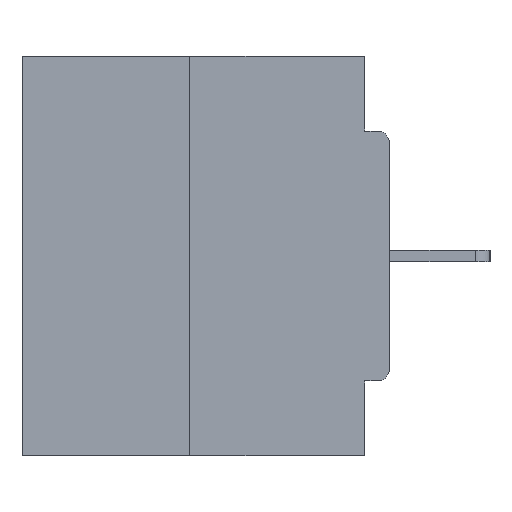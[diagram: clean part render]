
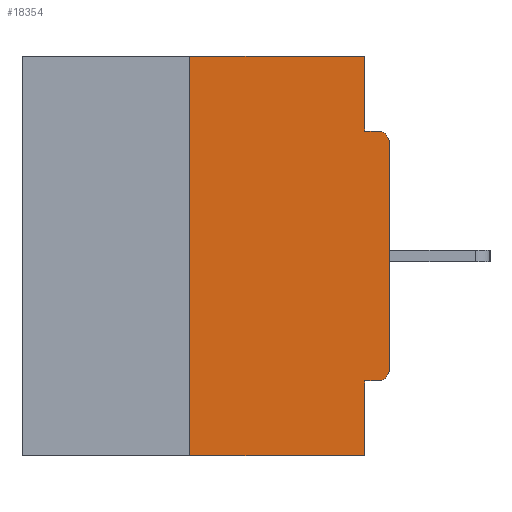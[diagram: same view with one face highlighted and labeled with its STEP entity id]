
A CAD part, left-side view. The second image highlights one B-rep face of the part: STEP entity #18354.
In plain terms, the highlighted planar face has unit normal (-1, 0, 0).
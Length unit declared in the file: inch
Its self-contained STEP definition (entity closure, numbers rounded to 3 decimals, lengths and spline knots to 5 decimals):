
#878 = CARTESIAN_POINT ( 'NONE',  ( 0., 0.25, -0.5 ) ) ;
#1514 = VERTEX_POINT ( 'NONE', #3295 ) ;
#1581 = VECTOR ( 'NONE', #13170, 39.37008 ) ;
#1629 = CARTESIAN_POINT ( 'NONE',  ( 0., 0.031, -0.5 ) ) ;
#2065 = LINE ( 'NONE', #14136, #22762 ) ;
#2434 = DIRECTION ( 'NONE',  ( 0., 1., 0. ) ) ;
#2832 = FACE_OUTER_BOUND ( 'NONE', #10365, .T. ) ;
#3229 = EDGE_CURVE ( 'NONE', #18467, #26430, #20417, .T. ) ;
#3295 = CARTESIAN_POINT ( 'NONE',  ( 0., 0.031, -0.0935 ) ) ;
#3951 = EDGE_CURVE ( 'NONE', #27794, #29450, #2065, .T. ) ;
#3990 = CARTESIAN_POINT ( 'NONE',  ( 0., 0., -0.3915 ) ) ;
#4044 = ORIENTED_EDGE ( 'NONE', *, *, #13576, .F. ) ;
#4891 = LINE ( 'NONE', #19871, #31558 ) ;
#5292 = DIRECTION ( 'NONE',  ( 0., 0., -1. ) ) ;
#5893 = CARTESIAN_POINT ( 'NONE',  ( 0., 0.46, 0. ) ) ;
#6233 = AXIS2_PLACEMENT_3D ( 'NONE', #11327, #23031, #31468 ) ;
#6636 = CARTESIAN_POINT ( 'NONE',  ( 0., 0., -0.0935 ) ) ;
#7240 = CARTESIAN_POINT ( 'NONE',  ( 0., 0., 0. ) ) ;
#8633 = VECTOR ( 'NONE', #35548, 39.37008 ) ;
#8899 = DIRECTION ( 'NONE',  ( 0., 0., -1. ) ) ;
#9162 = ORIENTED_EDGE ( 'NONE', *, *, #11961, .T. ) ;
#10341 = EDGE_CURVE ( 'NONE', #18789, #28685, #16888, .T. ) ;
#10365 = EDGE_LOOP ( 'NONE', ( #37006, #21003, #33109, #13666, #17884, #25788, #9162, #29178, #4044, #34429 ) ) ;
#11327 = CARTESIAN_POINT ( 'NONE',  ( 0., 0.015, -0.1085 ) ) ;
#11422 = VECTOR ( 'NONE', #18334, 39.37008 ) ;
#11650 = DIRECTION ( 'NONE',  ( 1., 0., 0. ) ) ;
#11884 = CARTESIAN_POINT ( 'NONE',  ( 0., 0.031, -0.5 ) ) ;
#11961 = EDGE_CURVE ( 'NONE', #14858, #30955, #36036, .T. ) ;
#12290 = CIRCLE ( 'NONE', #36192, 0.015 ) ;
#13170 = DIRECTION ( 'NONE',  ( 0., 0., 1. ) ) ;
#13576 = EDGE_CURVE ( 'NONE', #1514, #25197, #27536, .T. ) ;
#13666 = ORIENTED_EDGE ( 'NONE', *, *, #29842, .F. ) ;
#13844 = CARTESIAN_POINT ( 'NONE',  ( 0., 0.031, 0. ) ) ;
#14136 = CARTESIAN_POINT ( 'NONE',  ( 0., 0., -0.4065 ) ) ;
#14207 = VECTOR ( 'NONE', #23588, 39.37008 ) ;
#14349 = EDGE_CURVE ( 'NONE', #28685, #1514, #4891, .T. ) ;
#14858 = VERTEX_POINT ( 'NONE', #3990 ) ;
#15097 = DIRECTION ( 'NONE',  ( 0., 0., -1. ) ) ;
#15344 = EDGE_CURVE ( 'NONE', #18467, #18789, #36960, .T. ) ;
#16032 = CARTESIAN_POINT ( 'NONE',  ( 0., 0.25, 0. ) ) ;
#16495 = CARTESIAN_POINT ( 'NONE',  ( 0., 0.46, 0. ) ) ;
#16888 = LINE ( 'NONE', #16495, #33220 ) ;
#17884 = ORIENTED_EDGE ( 'NONE', *, *, #3951, .F. ) ;
#18334 = DIRECTION ( 'NONE',  ( 0., -1., 0. ) ) ;
#18354 = ADVANCED_FACE ( 'NONE', ( #2832 ), #26237, .F. ) ;
#18467 = VERTEX_POINT ( 'NONE', #878 ) ;
#18469 = CIRCLE ( 'NONE', #6233, 0.015 ) ;
#18789 = VERTEX_POINT ( 'NONE', #27075 ) ;
#19869 = VECTOR ( 'NONE', #27773, 39.37008 ) ;
#19871 = CARTESIAN_POINT ( 'NONE',  ( 0., 0.031, 0. ) ) ;
#20221 = DIRECTION ( 'NONE',  ( -1., 0., 0. ) ) ;
#20417 = LINE ( 'NONE', #37888, #8633 ) ;
#21003 = ORIENTED_EDGE ( 'NONE', *, *, #15344, .F. ) ;
#22442 = AXIS2_PLACEMENT_3D ( 'NONE', #5893, #11650, #15097 ) ;
#22762 = VECTOR ( 'NONE', #2434, 39.37008 ) ;
#22894 = EDGE_CURVE ( 'NONE', #27794, #14858, #12290, .T. ) ;
#23031 = DIRECTION ( 'NONE',  ( -1., 0., 0. ) ) ;
#23480 = CARTESIAN_POINT ( 'NONE',  ( 0., 0.015, -0.3915 ) ) ;
#23588 = DIRECTION ( 'NONE',  ( 0., 0., -1. ) ) ;
#25104 = EDGE_CURVE ( 'NONE', #30955, #25197, #18469, .T. ) ;
#25197 = VERTEX_POINT ( 'NONE', #35843 ) ;
#25788 = ORIENTED_EDGE ( 'NONE', *, *, #22894, .T. ) ;
#26237 = PLANE ( 'NONE',  #22442 ) ;
#26430 = VERTEX_POINT ( 'NONE', #1629 ) ;
#26459 = LINE ( 'NONE', #11884, #14207 ) ;
#27075 = CARTESIAN_POINT ( 'NONE',  ( 0., 0.25, 0. ) ) ;
#27536 = LINE ( 'NONE', #6636, #11422 ) ;
#27773 = DIRECTION ( 'NONE',  ( 0., 0., 1. ) ) ;
#27794 = VERTEX_POINT ( 'NONE', #28123 ) ;
#28123 = CARTESIAN_POINT ( 'NONE',  ( 0., 0.015, -0.4065 ) ) ;
#28685 = VERTEX_POINT ( 'NONE', #13844 ) ;
#29178 = ORIENTED_EDGE ( 'NONE', *, *, #25104, .T. ) ;
#29450 = VERTEX_POINT ( 'NONE', #31726 ) ;
#29842 = EDGE_CURVE ( 'NONE', #29450, #26430, #26459, .T. ) ;
#30955 = VERTEX_POINT ( 'NONE', #31950 ) ;
#31259 = DIRECTION ( 'NONE',  ( 0., -1., 0. ) ) ;
#31468 = DIRECTION ( 'NONE',  ( 0., 0., -1. ) ) ;
#31558 = VECTOR ( 'NONE', #5292, 39.37008 ) ;
#31726 = CARTESIAN_POINT ( 'NONE',  ( 0., 0.031, -0.4065 ) ) ;
#31950 = CARTESIAN_POINT ( 'NONE',  ( 0., 0., -0.1085 ) ) ;
#33109 = ORIENTED_EDGE ( 'NONE', *, *, #3229, .T. ) ;
#33220 = VECTOR ( 'NONE', #31259, 39.37008 ) ;
#34429 = ORIENTED_EDGE ( 'NONE', *, *, #14349, .F. ) ;
#35548 = DIRECTION ( 'NONE',  ( 0., -1., 0. ) ) ;
#35843 = CARTESIAN_POINT ( 'NONE',  ( 0., 0.015, -0.0935 ) ) ;
#36036 = LINE ( 'NONE', #7240, #19869 ) ;
#36192 = AXIS2_PLACEMENT_3D ( 'NONE', #23480, #20221, #8899 ) ;
#36960 = LINE ( 'NONE', #16032, #1581 ) ;
#37006 = ORIENTED_EDGE ( 'NONE', *, *, #10341, .F. ) ;
#37888 = CARTESIAN_POINT ( 'NONE',  ( 0., 0.46, -0.5 ) ) ;
